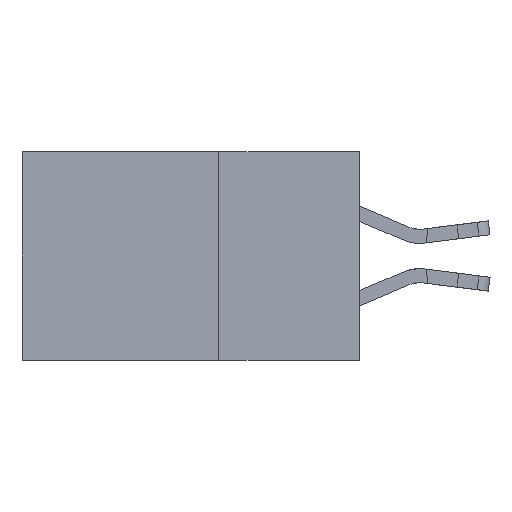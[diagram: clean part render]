
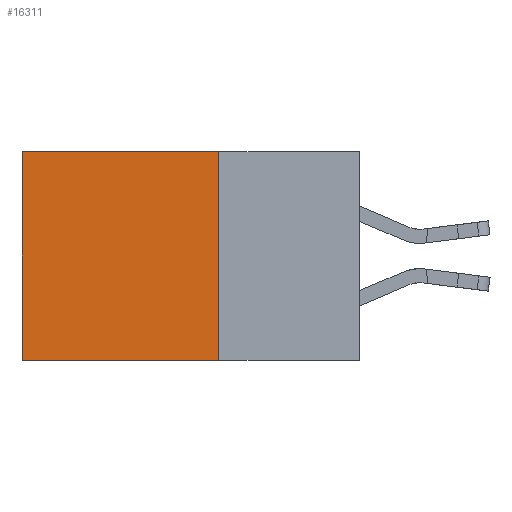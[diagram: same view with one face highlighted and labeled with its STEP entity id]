
A CAD part, left-side view. The second image highlights one B-rep face of the part: STEP entity #16311.
In plain terms, the highlighted planar face has unit normal (-1, 0, 0).
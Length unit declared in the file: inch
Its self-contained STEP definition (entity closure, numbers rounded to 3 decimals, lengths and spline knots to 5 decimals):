
#347 = ORIENTED_EDGE ( 'NONE', *, *, #32206, .F. ) ;
#1280 = AXIS2_PLACEMENT_3D ( 'NONE', #20768, #13064, #31416 ) ;
#1981 = DIRECTION ( 'NONE',  ( 0., 0., -1. ) ) ;
#2049 = EDGE_CURVE ( 'NONE', #9014, #2104, #29680, .T. ) ;
#2104 = VERTEX_POINT ( 'NONE', #5290 ) ;
#3674 = DIRECTION ( 'NONE',  ( 0., 0., -1. ) ) ;
#4767 = ORIENTED_EDGE ( 'NONE', *, *, #18274, .T. ) ;
#5174 = PLANE ( 'NONE',  #1280 ) ;
#5290 = CARTESIAN_POINT ( 'NONE',  ( 0.2875, 0.6, -0.37 ) ) ;
#6900 = LINE ( 'NONE', #33379, #22937 ) ;
#7454 = FACE_OUTER_BOUND ( 'NONE', #11070, .T. ) ;
#8050 = LINE ( 'NONE', #28464, #20740 ) ;
#9014 = VERTEX_POINT ( 'NONE', #21973 ) ;
#9219 = CARTESIAN_POINT ( 'NONE',  ( 0.2875, 0.25, -0.37 ) ) ;
#9854 = ORIENTED_EDGE ( 'NONE', *, *, #2049, .T. ) ;
#11070 = EDGE_LOOP ( 'NONE', ( #9854, #11770, #347, #4767 ) ) ;
#11128 = VERTEX_POINT ( 'NONE', #9219 ) ;
#11770 = ORIENTED_EDGE ( 'NONE', *, *, #21913, .F. ) ;
#12376 = DIRECTION ( 'NONE',  ( 0., 1., 0. ) ) ;
#13064 = DIRECTION ( 'NONE',  ( 1., 0., 0. ) ) ;
#13303 = VERTEX_POINT ( 'NONE', #29034 ) ;
#15255 = CARTESIAN_POINT ( 'NONE',  ( 0.2875, 0.25, 0. ) ) ;
#16311 = ADVANCED_FACE ( 'NONE', ( #7454 ), #5174, .F. ) ;
#18274 = EDGE_CURVE ( 'NONE', #13303, #9014, #29000, .T. ) ;
#20740 = VECTOR ( 'NONE', #21116, 39.37008 ) ;
#20768 = CARTESIAN_POINT ( 'NONE',  ( 0.2875, 0.25, 0. ) ) ;
#21116 = DIRECTION ( 'NONE',  ( 0., 1., 0. ) ) ;
#21913 = EDGE_CURVE ( 'NONE', #11128, #2104, #8050, .T. ) ;
#21973 = CARTESIAN_POINT ( 'NONE',  ( 0.2875, 0.6, 0. ) ) ;
#22937 = VECTOR ( 'NONE', #3674, 39.37008 ) ;
#23045 = CARTESIAN_POINT ( 'NONE',  ( 0.2875, 0.6, 0. ) ) ;
#24777 = VECTOR ( 'NONE', #12376, 39.37008 ) ;
#28460 = VECTOR ( 'NONE', #1981, 39.37008 ) ;
#28464 = CARTESIAN_POINT ( 'NONE',  ( 0.2875, 0.25, -0.37 ) ) ;
#29000 = LINE ( 'NONE', #15255, #24777 ) ;
#29034 = CARTESIAN_POINT ( 'NONE',  ( 0.2875, 0.25, 0. ) ) ;
#29680 = LINE ( 'NONE', #23045, #28460 ) ;
#31416 = DIRECTION ( 'NONE',  ( 0., 0., -1. ) ) ;
#32206 = EDGE_CURVE ( 'NONE', #13303, #11128, #6900, .T. ) ;
#33379 = CARTESIAN_POINT ( 'NONE',  ( 0.2875, 0.25, 0. ) ) ;
